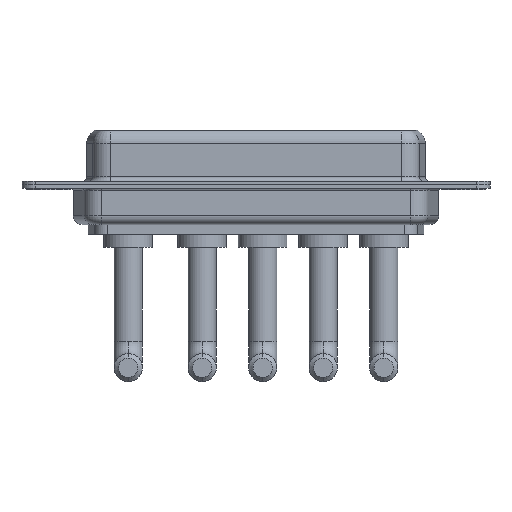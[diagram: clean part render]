
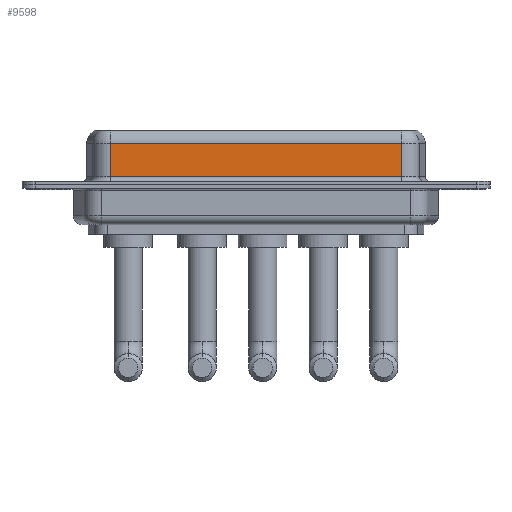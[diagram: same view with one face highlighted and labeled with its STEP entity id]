
A CAD part, front view. The second image highlights one B-rep face of the part: STEP entity #9598.
In plain terms, the highlighted planar face has unit normal (0, -1, 0).
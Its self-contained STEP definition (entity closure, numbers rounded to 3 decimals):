
#800 = ORIENTED_EDGE ( 'NONE', *, *, #5168, .T. ) ;
#858 = VERTEX_POINT ( 'NONE', #949 ) ;
#949 = CARTESIAN_POINT ( 'NONE',  ( 7.013, -3.95, 0.9 ) ) ;
#1692 = ORIENTED_EDGE ( 'NONE', *, *, #9739, .F. ) ;
#1815 = CARTESIAN_POINT ( 'NONE',  ( 40.037, -3.95, 6.4 ) ) ;
#1998 = VECTOR ( 'NONE', #7012, 1000. ) ;
#2099 = CARTESIAN_POINT ( 'NONE',  ( 40.037, -3.95, 6.4 ) ) ;
#2810 = FACE_OUTER_BOUND ( 'NONE', #3394, .T. ) ;
#3003 = VERTEX_POINT ( 'NONE', #4331 ) ;
#3223 = CARTESIAN_POINT ( 'NONE',  ( 40.037, -3.95, 4.65 ) ) ;
#3394 = EDGE_LOOP ( 'NONE', ( #1692, #800, #9700, #5754 ) ) ;
#3410 = DIRECTION ( 'NONE',  ( 0., 0., -1. ) ) ;
#3736 = EDGE_CURVE ( 'NONE', #858, #3003, #8046, .T. ) ;
#3743 = AXIS2_PLACEMENT_3D ( 'NONE', #2099, #7064, #3744 ) ;
#3744 = DIRECTION ( 'NONE',  ( 0., 0., 1. ) ) ;
#3836 = DIRECTION ( 'NONE',  ( 1., 0., 0. ) ) ;
#4104 = LINE ( 'NONE', #3223, #10876 ) ;
#4134 = CARTESIAN_POINT ( 'NONE',  ( 40.037, -3.95, 4.65 ) ) ;
#4331 = CARTESIAN_POINT ( 'NONE',  ( 40.037, -3.95, 0.9 ) ) ;
#5168 = EDGE_CURVE ( 'NONE', #9784, #9660, #4104, .T. ) ;
#5396 = CARTESIAN_POINT ( 'NONE',  ( 7.013, -3.95, 6.4 ) ) ;
#5754 = ORIENTED_EDGE ( 'NONE', *, *, #3736, .T. ) ;
#6324 = CARTESIAN_POINT ( 'NONE',  ( 40.037, -3.95, 0.9 ) ) ;
#6588 = DIRECTION ( 'NONE',  ( -1., 0., 0. ) ) ;
#6887 = VECTOR ( 'NONE', #3836, 1000. ) ;
#7012 = DIRECTION ( 'NONE',  ( 0., 0., -1. ) ) ;
#7064 = DIRECTION ( 'NONE',  ( 0., 1., 0. ) ) ;
#7996 = VECTOR ( 'NONE', #3410, 1000. ) ;
#8005 = LINE ( 'NONE', #5396, #1998 ) ;
#8046 = LINE ( 'NONE', #6324, #6887 ) ;
#8237 = CARTESIAN_POINT ( 'NONE',  ( 7.013, -3.95, 4.65 ) ) ;
#9447 = EDGE_CURVE ( 'NONE', #9660, #858, #8005, .T. ) ;
#9569 = PLANE ( 'NONE',  #3743 ) ;
#9598 = ADVANCED_FACE ( 'NONE', ( #2810 ), #9569, .F. ) ;
#9660 = VERTEX_POINT ( 'NONE', #8237 ) ;
#9700 = ORIENTED_EDGE ( 'NONE', *, *, #9447, .T. ) ;
#9739 = EDGE_CURVE ( 'NONE', #9784, #3003, #10895, .T. ) ;
#9784 = VERTEX_POINT ( 'NONE', #4134 ) ;
#10876 = VECTOR ( 'NONE', #6588, 1000. ) ;
#10895 = LINE ( 'NONE', #1815, #7996 ) ;
